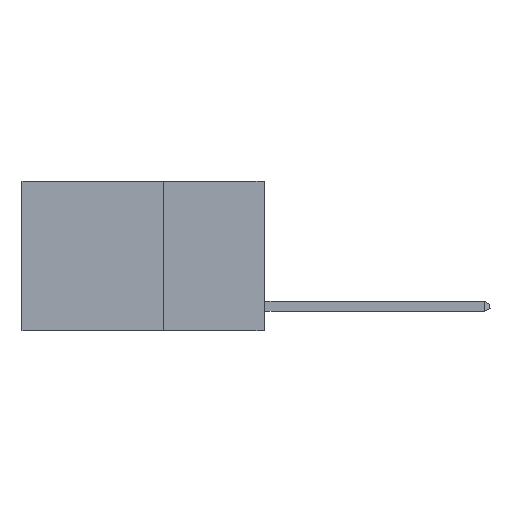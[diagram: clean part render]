
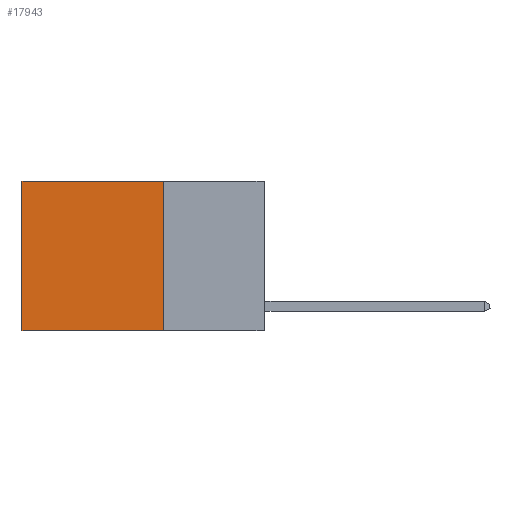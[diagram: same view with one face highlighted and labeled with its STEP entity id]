
A CAD part, left-side view. The second image highlights one B-rep face of the part: STEP entity #17943.
In plain terms, the highlighted planar face has unit normal (-1, 0, 0).
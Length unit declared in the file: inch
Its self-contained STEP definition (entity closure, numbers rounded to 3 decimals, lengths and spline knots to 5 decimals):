
#79 = FACE_OUTER_BOUND ( 'NONE', #11544, .T. ) ;
#266 = LINE ( 'NONE', #21414, #17255 ) ;
#514 = CARTESIAN_POINT ( 'NONE',  ( 0.2625, 0.25, 0. ) ) ;
#2736 = PLANE ( 'NONE',  #5927 ) ;
#4585 = VECTOR ( 'NONE', #12738, 39.37008 ) ;
#4599 = VERTEX_POINT ( 'NONE', #26754 ) ;
#4961 = DIRECTION ( 'NONE',  ( 0., 0., -1. ) ) ;
#5025 = EDGE_CURVE ( 'NONE', #4599, #23082, #11173, .T. ) ;
#5351 = VECTOR ( 'NONE', #22438, 39.37008 ) ;
#5466 = CARTESIAN_POINT ( 'NONE',  ( 0.2625, 0.25, 0. ) ) ;
#5927 = AXIS2_PLACEMENT_3D ( 'NONE', #514, #9437, #24949 ) ;
#6060 = LINE ( 'NONE', #17990, #5351 ) ;
#8736 = EDGE_CURVE ( 'NONE', #18772, #20533, #26521, .T. ) ;
#9437 = DIRECTION ( 'NONE',  ( 1., 0., 0. ) ) ;
#9950 = ORIENTED_EDGE ( 'NONE', *, *, #27668, .T. ) ;
#10749 = CARTESIAN_POINT ( 'NONE',  ( 0.2625, 0.25, -0.37 ) ) ;
#11173 = LINE ( 'NONE', #14898, #4585 ) ;
#11544 = EDGE_LOOP ( 'NONE', ( #25284, #19276, #13064, #9950 ) ) ;
#12482 = EDGE_CURVE ( 'NONE', #20533, #23082, #266, .T. ) ;
#12738 = DIRECTION ( 'NONE',  ( 0., 0., -1. ) ) ;
#13064 = ORIENTED_EDGE ( 'NONE', *, *, #8736, .F. ) ;
#14898 = CARTESIAN_POINT ( 'NONE',  ( 0.2625, 0.6, 0. ) ) ;
#16044 = CARTESIAN_POINT ( 'NONE',  ( 0.2625, 0.25, 0. ) ) ;
#17255 = VECTOR ( 'NONE', #28076, 39.37008 ) ;
#17943 = ADVANCED_FACE ( 'NONE', ( #79 ), #2736, .F. ) ;
#17990 = CARTESIAN_POINT ( 'NONE',  ( 0.2625, 0.25, 0. ) ) ;
#18772 = VERTEX_POINT ( 'NONE', #5466 ) ;
#19271 = VECTOR ( 'NONE', #4961, 39.37008 ) ;
#19276 = ORIENTED_EDGE ( 'NONE', *, *, #12482, .F. ) ;
#20533 = VERTEX_POINT ( 'NONE', #10749 ) ;
#21414 = CARTESIAN_POINT ( 'NONE',  ( 0.2625, 0.25, -0.37 ) ) ;
#21461 = CARTESIAN_POINT ( 'NONE',  ( 0.2625, 0.6, -0.37 ) ) ;
#22438 = DIRECTION ( 'NONE',  ( 0., 1., 0. ) ) ;
#23082 = VERTEX_POINT ( 'NONE', #21461 ) ;
#24949 = DIRECTION ( 'NONE',  ( 0., 0., -1. ) ) ;
#25284 = ORIENTED_EDGE ( 'NONE', *, *, #5025, .T. ) ;
#26521 = LINE ( 'NONE', #16044, #19271 ) ;
#26754 = CARTESIAN_POINT ( 'NONE',  ( 0.2625, 0.6, 0. ) ) ;
#27668 = EDGE_CURVE ( 'NONE', #18772, #4599, #6060, .T. ) ;
#28076 = DIRECTION ( 'NONE',  ( 0., 1., 0. ) ) ;
